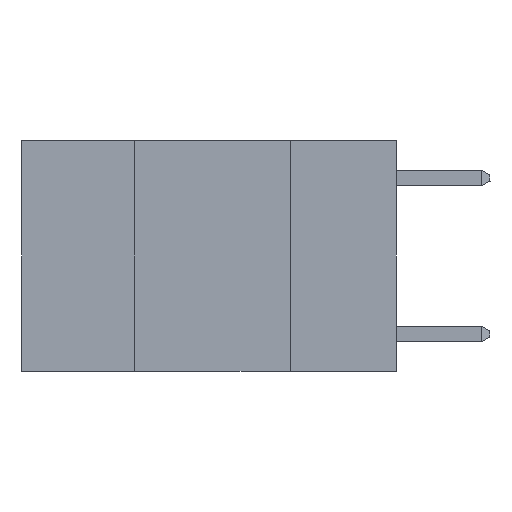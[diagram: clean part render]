
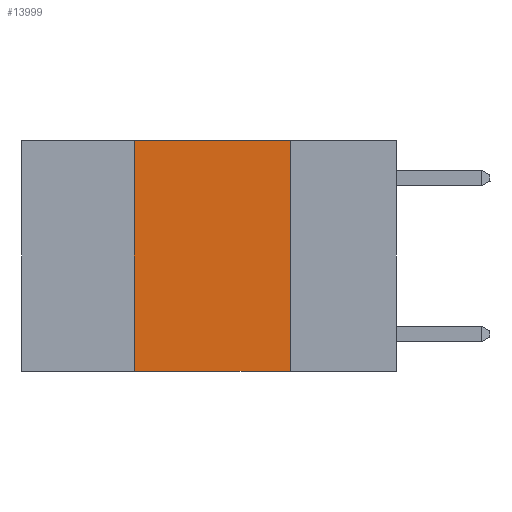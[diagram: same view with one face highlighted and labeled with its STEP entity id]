
A CAD part, left-side view. The second image highlights one B-rep face of the part: STEP entity #13999.
In plain terms, the highlighted planar face has unit normal (-1, 0, 0).
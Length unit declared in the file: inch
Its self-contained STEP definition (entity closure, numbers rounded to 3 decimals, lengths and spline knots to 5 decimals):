
#104 = ORIENTED_EDGE ( 'NONE', *, *, #8674, .F. ) ;
#988 = LINE ( 'NONE', #9250, #3005 ) ;
#1273 = DIRECTION ( 'NONE',  ( 0., 0., -1. ) ) ;
#1304 = DIRECTION ( 'NONE',  ( 0., 0., 1. ) ) ;
#1550 = ORIENTED_EDGE ( 'NONE', *, *, #5430, .F. ) ;
#2087 = VERTEX_POINT ( 'NONE', #17221 ) ;
#2156 = EDGE_CURVE ( 'NONE', #2087, #3263, #988, .T. ) ;
#2481 = AXIS2_PLACEMENT_3D ( 'NONE', #11013, #13727, #5485 ) ;
#2774 = FACE_OUTER_BOUND ( 'NONE', #9028, .T. ) ;
#3005 = VECTOR ( 'NONE', #14847, 39.37008 ) ;
#3263 = VERTEX_POINT ( 'NONE', #9333 ) ;
#4504 = VERTEX_POINT ( 'NONE', #12898 ) ;
#4955 = CARTESIAN_POINT ( 'NONE',  ( 0., 0.6, 0. ) ) ;
#5395 = PLANE ( 'NONE',  #2481 ) ;
#5430 = EDGE_CURVE ( 'NONE', #2087, #13039, #10218, .T. ) ;
#5485 = DIRECTION ( 'NONE',  ( 0., 0., -1. ) ) ;
#8674 = EDGE_CURVE ( 'NONE', #13039, #4504, #10210, .T. ) ;
#9028 = EDGE_LOOP ( 'NONE', ( #10427, #104, #1550, #12223 ) ) ;
#9250 = CARTESIAN_POINT ( 'NONE',  ( 0., 0.6, -0.37 ) ) ;
#9333 = CARTESIAN_POINT ( 'NONE',  ( 0., 0.17, -0.37 ) ) ;
#10210 = LINE ( 'NONE', #4955, #16477 ) ;
#10218 = LINE ( 'NONE', #14892, #15927 ) ;
#10427 = ORIENTED_EDGE ( 'NONE', *, *, #14973, .F. ) ;
#10972 = CARTESIAN_POINT ( 'NONE',  ( 0., 0.17, 0. ) ) ;
#11013 = CARTESIAN_POINT ( 'NONE',  ( 0., 0.6, 0. ) ) ;
#11809 = CARTESIAN_POINT ( 'NONE',  ( 0., 0.42, 0. ) ) ;
#11816 = DIRECTION ( 'NONE',  ( 0., -1., 0. ) ) ;
#12223 = ORIENTED_EDGE ( 'NONE', *, *, #2156, .T. ) ;
#12898 = CARTESIAN_POINT ( 'NONE',  ( 0., 0.17, 0. ) ) ;
#13039 = VERTEX_POINT ( 'NONE', #11809 ) ;
#13214 = VECTOR ( 'NONE', #1273, 39.37008 ) ;
#13727 = DIRECTION ( 'NONE',  ( 1., 0., 0. ) ) ;
#13999 = ADVANCED_FACE ( 'NONE', ( #2774 ), #5395, .F. ) ;
#14847 = DIRECTION ( 'NONE',  ( 0., -1., 0. ) ) ;
#14892 = CARTESIAN_POINT ( 'NONE',  ( 0., 0.42, 0. ) ) ;
#14973 = EDGE_CURVE ( 'NONE', #4504, #3263, #17573, .T. ) ;
#15927 = VECTOR ( 'NONE', #1304, 39.37008 ) ;
#16477 = VECTOR ( 'NONE', #11816, 39.37008 ) ;
#17221 = CARTESIAN_POINT ( 'NONE',  ( 0., 0.42, -0.37 ) ) ;
#17573 = LINE ( 'NONE', #10972, #13214 ) ;
